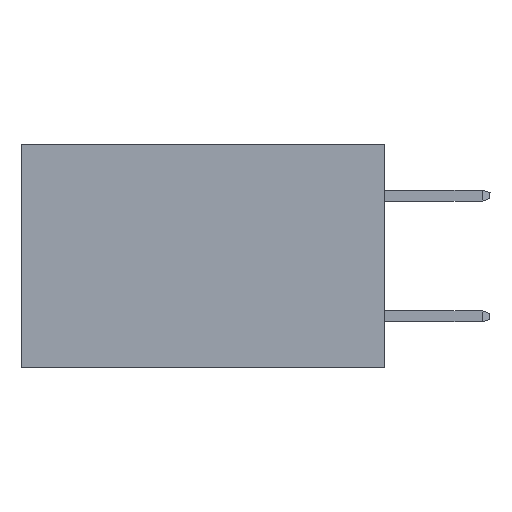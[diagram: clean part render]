
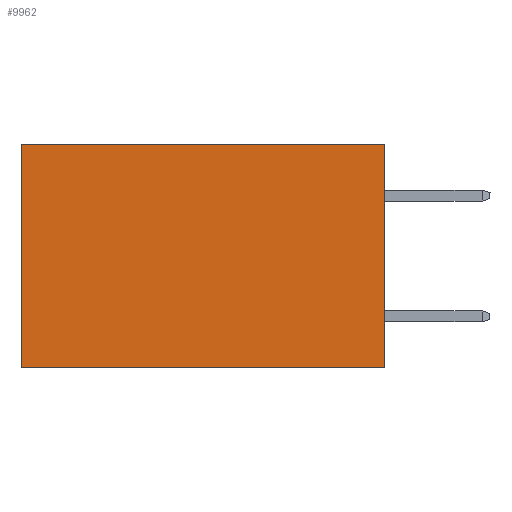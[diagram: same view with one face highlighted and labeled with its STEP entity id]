
A CAD part, left-side view. The second image highlights one B-rep face of the part: STEP entity #9962.
In plain terms, the highlighted planar face has unit normal (-1, 0, 0).
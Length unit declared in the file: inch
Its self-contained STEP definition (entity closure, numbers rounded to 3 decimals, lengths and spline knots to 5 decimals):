
#1156 = ORIENTED_EDGE ( 'NONE', *, *, #14991, .F. ) ;
#1309 = ORIENTED_EDGE ( 'NONE', *, *, #15041, .T. ) ;
#1748 = CARTESIAN_POINT ( 'NONE',  ( 0.298, 0.6, 0. ) ) ;
#1953 = LINE ( 'NONE', #13740, #17620 ) ;
#2508 = DIRECTION ( 'NONE',  ( 0., 1., 0. ) ) ;
#2923 = FACE_OUTER_BOUND ( 'NONE', #7520, .T. ) ;
#3435 = CARTESIAN_POINT ( 'NONE',  ( 0.298, 0., 0. ) ) ;
#3625 = EDGE_CURVE ( 'NONE', #12043, #5284, #4037, .T. ) ;
#3633 = DIRECTION ( 'NONE',  ( 0., 0., -1. ) ) ;
#4037 = LINE ( 'NONE', #8029, #5224 ) ;
#4501 = CARTESIAN_POINT ( 'NONE',  ( 0.298, 0.6, 0. ) ) ;
#5224 = VECTOR ( 'NONE', #2508, 39.37008 ) ;
#5284 = VERTEX_POINT ( 'NONE', #4501 ) ;
#5354 = VECTOR ( 'NONE', #3633, 39.37008 ) ;
#5589 = EDGE_CURVE ( 'NONE', #18299, #18185, #1953, .T. ) ;
#5624 = VECTOR ( 'NONE', #20480, 39.37008 ) ;
#7373 = LINE ( 'NONE', #11102, #5624 ) ;
#7520 = EDGE_LOOP ( 'NONE', ( #1309, #12844, #1156, #9235 ) ) ;
#7640 = CARTESIAN_POINT ( 'NONE',  ( 0.298, 0.6, -0.37 ) ) ;
#7671 = AXIS2_PLACEMENT_3D ( 'NONE', #11898, #21301, #19465 ) ;
#8029 = CARTESIAN_POINT ( 'NONE',  ( 0.298, 0., 0. ) ) ;
#9235 = ORIENTED_EDGE ( 'NONE', *, *, #3625, .T. ) ;
#9962 = ADVANCED_FACE ( 'NONE', ( #2923 ), #12217, .F. ) ;
#11102 = CARTESIAN_POINT ( 'NONE',  ( 0.298, 0., 0. ) ) ;
#11898 = CARTESIAN_POINT ( 'NONE',  ( 0.298, 0., 0. ) ) ;
#12043 = VERTEX_POINT ( 'NONE', #3435 ) ;
#12217 = PLANE ( 'NONE',  #7671 ) ;
#12844 = ORIENTED_EDGE ( 'NONE', *, *, #5589, .F. ) ;
#13740 = CARTESIAN_POINT ( 'NONE',  ( 0.298, 0., -0.37 ) ) ;
#14611 = LINE ( 'NONE', #1748, #5354 ) ;
#14991 = EDGE_CURVE ( 'NONE', #12043, #18299, #7373, .T. ) ;
#15041 = EDGE_CURVE ( 'NONE', #5284, #18185, #14611, .T. ) ;
#17445 = DIRECTION ( 'NONE',  ( 0., 1., 0. ) ) ;
#17620 = VECTOR ( 'NONE', #17445, 39.37008 ) ;
#18185 = VERTEX_POINT ( 'NONE', #7640 ) ;
#18299 = VERTEX_POINT ( 'NONE', #22003 ) ;
#19465 = DIRECTION ( 'NONE',  ( 0., 0., -1. ) ) ;
#20480 = DIRECTION ( 'NONE',  ( 0., 0., -1. ) ) ;
#21301 = DIRECTION ( 'NONE',  ( 1., 0., 0. ) ) ;
#22003 = CARTESIAN_POINT ( 'NONE',  ( 0.298, 0., -0.37 ) ) ;
